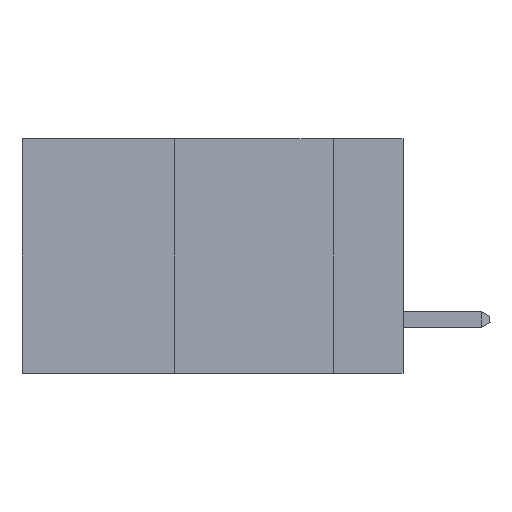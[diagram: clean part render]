
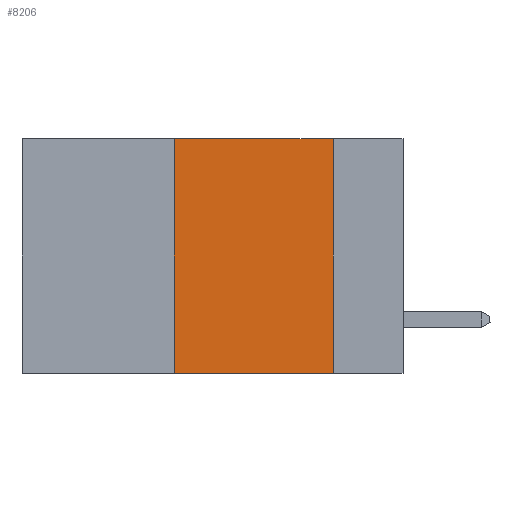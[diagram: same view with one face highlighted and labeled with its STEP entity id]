
A CAD part, left-side view. The second image highlights one B-rep face of the part: STEP entity #8206.
In plain terms, the highlighted planar face has unit normal (-1, 0, 0).
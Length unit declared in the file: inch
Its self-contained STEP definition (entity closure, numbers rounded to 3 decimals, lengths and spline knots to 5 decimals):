
#621 = VERTEX_POINT ( 'NONE', #6870 ) ;
#1271 = PLANE ( 'NONE',  #5147 ) ;
#1621 = DIRECTION ( 'NONE',  ( 0., 0., -1. ) ) ;
#1677 = CARTESIAN_POINT ( 'NONE',  ( 0., 0.11, 0. ) ) ;
#1709 = CARTESIAN_POINT ( 'NONE',  ( 0., 0.6, 0. ) ) ;
#1723 = ORIENTED_EDGE ( 'NONE', *, *, #4539, .F. ) ;
#3076 = VERTEX_POINT ( 'NONE', #16364 ) ;
#3910 = DIRECTION ( 'NONE',  ( 1., 0., 0. ) ) ;
#4173 = CARTESIAN_POINT ( 'NONE',  ( 0., 0.36, 0. ) ) ;
#4539 = EDGE_CURVE ( 'NONE', #3076, #7289, #8592, .T. ) ;
#4742 = VERTEX_POINT ( 'NONE', #6235 ) ;
#5147 = AXIS2_PLACEMENT_3D ( 'NONE', #13353, #3910, #12001 ) ;
#6235 = CARTESIAN_POINT ( 'NONE',  ( 0., 0.36, -0.37 ) ) ;
#6370 = EDGE_CURVE ( 'NONE', #4742, #3076, #6431, .T. ) ;
#6431 = LINE ( 'NONE', #4173, #9168 ) ;
#6517 = CARTESIAN_POINT ( 'NONE',  ( 0., 0.6, -0.37 ) ) ;
#6870 = CARTESIAN_POINT ( 'NONE',  ( 0., 0.11, -0.37 ) ) ;
#7289 = VERTEX_POINT ( 'NONE', #10682 ) ;
#7312 = LINE ( 'NONE', #6517, #16209 ) ;
#8043 = ORIENTED_EDGE ( 'NONE', *, *, #11392, .T. ) ;
#8206 = ADVANCED_FACE ( 'NONE', ( #8482 ), #1271, .F. ) ;
#8482 = FACE_OUTER_BOUND ( 'NONE', #12473, .T. ) ;
#8592 = LINE ( 'NONE', #1709, #13246 ) ;
#9168 = VECTOR ( 'NONE', #13680, 39.37008 ) ;
#10492 = DIRECTION ( 'NONE',  ( 0., -1., 0. ) ) ;
#10682 = CARTESIAN_POINT ( 'NONE',  ( 0., 0.11, 0. ) ) ;
#10753 = VECTOR ( 'NONE', #1621, 39.37008 ) ;
#11392 = EDGE_CURVE ( 'NONE', #4742, #621, #7312, .T. ) ;
#12001 = DIRECTION ( 'NONE',  ( 0., 0., -1. ) ) ;
#12473 = EDGE_LOOP ( 'NONE', ( #15371, #1723, #15801, #8043 ) ) ;
#13050 = LINE ( 'NONE', #1677, #10753 ) ;
#13246 = VECTOR ( 'NONE', #13875, 39.37008 ) ;
#13353 = CARTESIAN_POINT ( 'NONE',  ( 0., 0.6, 0. ) ) ;
#13680 = DIRECTION ( 'NONE',  ( 0., 0., 1. ) ) ;
#13875 = DIRECTION ( 'NONE',  ( 0., -1., 0. ) ) ;
#15068 = EDGE_CURVE ( 'NONE', #7289, #621, #13050, .T. ) ;
#15371 = ORIENTED_EDGE ( 'NONE', *, *, #15068, .F. ) ;
#15801 = ORIENTED_EDGE ( 'NONE', *, *, #6370, .F. ) ;
#16209 = VECTOR ( 'NONE', #10492, 39.37008 ) ;
#16364 = CARTESIAN_POINT ( 'NONE',  ( 0., 0.36, 0. ) ) ;
